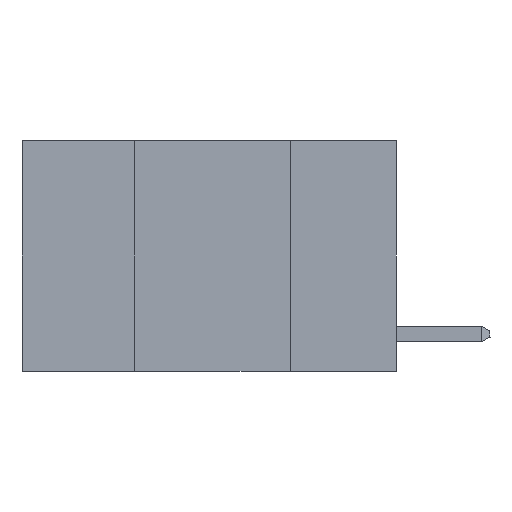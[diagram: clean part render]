
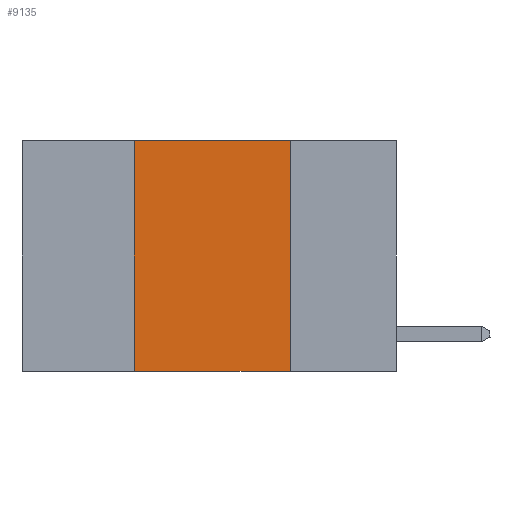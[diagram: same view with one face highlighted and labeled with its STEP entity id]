
A CAD part, left-side view. The second image highlights one B-rep face of the part: STEP entity #9135.
In plain terms, the highlighted planar face has unit normal (-1, 0, 0).
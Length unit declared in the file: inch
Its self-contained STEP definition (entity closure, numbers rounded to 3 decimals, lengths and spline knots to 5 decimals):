
#335 = VERTEX_POINT ( 'NONE', #4693 ) ;
#882 = ORIENTED_EDGE ( 'NONE', *, *, #15162, .F. ) ;
#1137 = ORIENTED_EDGE ( 'NONE', *, *, #15221, .T. ) ;
#1659 = VECTOR ( 'NONE', #12607, 39.37008 ) ;
#1870 = FACE_OUTER_BOUND ( 'NONE', #13467, .T. ) ;
#2832 = AXIS2_PLACEMENT_3D ( 'NONE', #12405, #5707, #17492 ) ;
#3631 = ORIENTED_EDGE ( 'NONE', *, *, #7941, .F. ) ;
#4340 = DIRECTION ( 'NONE',  ( 0., -1., 0. ) ) ;
#4367 = ORIENTED_EDGE ( 'NONE', *, *, #14607, .F. ) ;
#4392 = VERTEX_POINT ( 'NONE', #10000 ) ;
#4693 = CARTESIAN_POINT ( 'NONE',  ( 0., 0.17, 0. ) ) ;
#5707 = DIRECTION ( 'NONE',  ( 1., 0., 0. ) ) ;
#5841 = DIRECTION ( 'NONE',  ( 0., -1., 0. ) ) ;
#5897 = VECTOR ( 'NONE', #4340, 39.37008 ) ;
#6430 = LINE ( 'NONE', #7688, #5897 ) ;
#7015 = VERTEX_POINT ( 'NONE', #14796 ) ;
#7360 = CARTESIAN_POINT ( 'NONE',  ( 0., 0.17, 0. ) ) ;
#7688 = CARTESIAN_POINT ( 'NONE',  ( 0., 0.6, 0. ) ) ;
#7941 = EDGE_CURVE ( 'NONE', #7015, #15468, #15083, .T. ) ;
#9003 = PLANE ( 'NONE',  #2832 ) ;
#9135 = ADVANCED_FACE ( 'NONE', ( #1870 ), #9003, .F. ) ;
#9879 = CARTESIAN_POINT ( 'NONE',  ( 0., 0.42, 0. ) ) ;
#10000 = CARTESIAN_POINT ( 'NONE',  ( 0., 0.17, -0.37 ) ) ;
#10767 = DIRECTION ( 'NONE',  ( 0., 0., -1. ) ) ;
#12198 = VECTOR ( 'NONE', #10767, 39.37008 ) ;
#12405 = CARTESIAN_POINT ( 'NONE',  ( 0., 0.6, 0. ) ) ;
#12607 = DIRECTION ( 'NONE',  ( 0., 0., 1. ) ) ;
#13467 = EDGE_LOOP ( 'NONE', ( #882, #4367, #3631, #1137 ) ) ;
#14607 = EDGE_CURVE ( 'NONE', #15468, #335, #6430, .T. ) ;
#14796 = CARTESIAN_POINT ( 'NONE',  ( 0., 0.42, -0.37 ) ) ;
#15083 = LINE ( 'NONE', #17619, #1659 ) ;
#15162 = EDGE_CURVE ( 'NONE', #335, #4392, #16682, .T. ) ;
#15221 = EDGE_CURVE ( 'NONE', #7015, #4392, #20117, .T. ) ;
#15468 = VERTEX_POINT ( 'NONE', #9879 ) ;
#16682 = LINE ( 'NONE', #7360, #12198 ) ;
#17492 = DIRECTION ( 'NONE',  ( 0., 0., -1. ) ) ;
#17619 = CARTESIAN_POINT ( 'NONE',  ( 0., 0.42, 0. ) ) ;
#19311 = CARTESIAN_POINT ( 'NONE',  ( 0., 0.6, -0.37 ) ) ;
#19576 = VECTOR ( 'NONE', #5841, 39.37008 ) ;
#20117 = LINE ( 'NONE', #19311, #19576 ) ;
